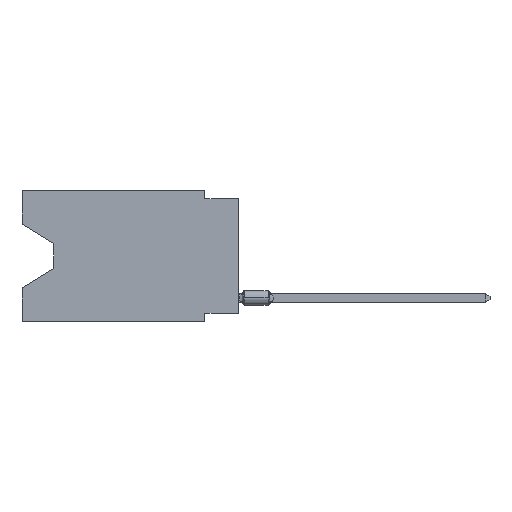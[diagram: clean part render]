
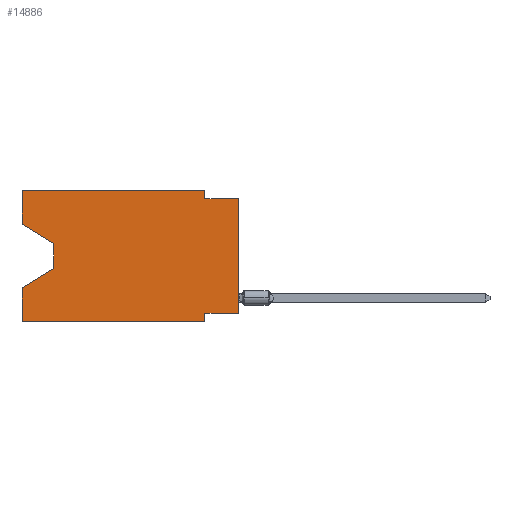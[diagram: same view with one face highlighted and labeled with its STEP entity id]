
A CAD part, left-side view. The second image highlights one B-rep face of the part: STEP entity #14886.
In plain terms, the highlighted planar face has unit normal (-1, 0, 0).
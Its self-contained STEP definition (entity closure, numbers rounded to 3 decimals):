
#68 = CARTESIAN_POINT ( 'NONE',  ( 0., 16.383, 0. ) ) ;
#351 = ORIENTED_EDGE ( 'NONE', *, *, #17122, .T. ) ;
#352 = DIRECTION ( 'NONE',  ( 0., -1., 0. ) ) ;
#699 = DIRECTION ( 'NONE',  ( 1., 0., 0. ) ) ;
#1004 = LINE ( 'NONE', #1097, #1624 ) ;
#1097 = CARTESIAN_POINT ( 'NONE',  ( 0., 2.54, 0. ) ) ;
#1304 = CARTESIAN_POINT ( 'NONE',  ( 0., 16.383, -2.546 ) ) ;
#1529 = CARTESIAN_POINT ( 'NONE',  ( 0., 2.54, -9.271 ) ) ;
#1624 = VECTOR ( 'NONE', #12020, 1000. ) ;
#1640 = CARTESIAN_POINT ( 'NONE',  ( 0., 0., -9.271 ) ) ;
#2040 = LINE ( 'NONE', #15904, #15193 ) ;
#2059 = VERTEX_POINT ( 'NONE', #4552 ) ;
#2344 = CARTESIAN_POINT ( 'NONE',  ( 0., 13.97, -5.893 ) ) ;
#2637 = VERTEX_POINT ( 'NONE', #11923 ) ;
#2653 = DIRECTION ( 'NONE',  ( 0., 0., 1. ) ) ;
#2704 = CARTESIAN_POINT ( 'NONE',  ( 0., 13.97, -5.893 ) ) ;
#2888 = VECTOR ( 'NONE', #3939, 1000. ) ;
#2911 = VERTEX_POINT ( 'NONE', #11266 ) ;
#3112 = EDGE_CURVE ( 'NONE', #11366, #15865, #9222, .T. ) ;
#3512 = VECTOR ( 'NONE', #2653, 1000. ) ;
#3543 = LINE ( 'NONE', #2344, #10102 ) ;
#3648 = ORIENTED_EDGE ( 'NONE', *, *, #13792, .T. ) ;
#3939 = DIRECTION ( 'NONE',  ( 0., 0., -1. ) ) ;
#4046 = CARTESIAN_POINT ( 'NONE',  ( 0., 0., 0. ) ) ;
#4280 = EDGE_CURVE ( 'NONE', #17562, #2059, #11277, .T. ) ;
#4552 = CARTESIAN_POINT ( 'NONE',  ( 0., 2.54, 0. ) ) ;
#4559 = VECTOR ( 'NONE', #352, 1000. ) ;
#4783 = EDGE_CURVE ( 'NONE', #11562, #2637, #3543, .T. ) ;
#5107 = VECTOR ( 'NONE', #10067, 1000. ) ;
#5238 = PLANE ( 'NONE',  #9570 ) ;
#5374 = LINE ( 'NONE', #1304, #11021 ) ;
#5442 = CARTESIAN_POINT ( 'NONE',  ( 0., 0., -0.635 ) ) ;
#5646 = VECTOR ( 'NONE', #7770, 1000. ) ;
#6226 = DIRECTION ( 'NONE',  ( 0., 0.855, -0.519 ) ) ;
#6494 = VERTEX_POINT ( 'NONE', #14141 ) ;
#6963 = EDGE_CURVE ( 'NONE', #7016, #17491, #8126, .T. ) ;
#7016 = VERTEX_POINT ( 'NONE', #1640 ) ;
#7262 = VECTOR ( 'NONE', #18008, 1000. ) ;
#7550 = ORIENTED_EDGE ( 'NONE', *, *, #3112, .F. ) ;
#7770 = DIRECTION ( 'NONE',  ( 0., -1., 0. ) ) ;
#8126 = LINE ( 'NONE', #4046, #7262 ) ;
#8236 = ORIENTED_EDGE ( 'NONE', *, *, #13847, .F. ) ;
#8739 = VERTEX_POINT ( 'NONE', #11519 ) ;
#8771 = ORIENTED_EDGE ( 'NONE', *, *, #13661, .F. ) ;
#9021 = EDGE_LOOP ( 'NONE', ( #351, #3648, #15853, #8771, #10507, #7550, #16704, #13132, #16457, #8236, #15598, #14436 ) ) ;
#9061 = LINE ( 'NONE', #14797, #4559 ) ;
#9222 = LINE ( 'NONE', #9313, #2888 ) ;
#9313 = CARTESIAN_POINT ( 'NONE',  ( 0., 2.54, -9.906 ) ) ;
#9332 = CARTESIAN_POINT ( 'NONE',  ( 0., 13.97, -4.013 ) ) ;
#9506 = LINE ( 'NONE', #9332, #14004 ) ;
#9570 = AXIS2_PLACEMENT_3D ( 'NONE', #11996, #699, #10512 ) ;
#9881 = LINE ( 'NONE', #14230, #14879 ) ;
#10067 = DIRECTION ( 'NONE',  ( 0., -1., 0. ) ) ;
#10102 = VECTOR ( 'NONE', #6226, 1000. ) ;
#10199 = EDGE_CURVE ( 'NONE', #2911, #17562, #16982, .T. ) ;
#10507 = ORIENTED_EDGE ( 'NONE', *, *, #13649, .T. ) ;
#10512 = DIRECTION ( 'NONE',  ( 0., 0., -1. ) ) ;
#10697 = FACE_OUTER_BOUND ( 'NONE', #9021, .T. ) ;
#10812 = DIRECTION ( 'NONE',  ( 0., 0., -1. ) ) ;
#10987 = CARTESIAN_POINT ( 'NONE',  ( 0., 2.54, -9.906 ) ) ;
#11019 = DIRECTION ( 'NONE',  ( 0., -0.855, -0.519 ) ) ;
#11021 = VECTOR ( 'NONE', #11019, 1000. ) ;
#11266 = CARTESIAN_POINT ( 'NONE',  ( 0., 16.383, -2.546 ) ) ;
#11277 = LINE ( 'NONE', #15624, #5107 ) ;
#11366 = VERTEX_POINT ( 'NONE', #1529 ) ;
#11507 = VERTEX_POINT ( 'NONE', #12151 ) ;
#11519 = CARTESIAN_POINT ( 'NONE',  ( 0., 2.54, -0.635 ) ) ;
#11562 = VERTEX_POINT ( 'NONE', #2704 ) ;
#11923 = CARTESIAN_POINT ( 'NONE',  ( 0., 16.383, -7.36 ) ) ;
#11996 = CARTESIAN_POINT ( 'NONE',  ( 0., 16.383, 0. ) ) ;
#12020 = DIRECTION ( 'NONE',  ( 0., 0., -1. ) ) ;
#12151 = CARTESIAN_POINT ( 'NONE',  ( 0., 16.383, -9.906 ) ) ;
#12233 = EDGE_CURVE ( 'NONE', #8739, #17491, #14605, .T. ) ;
#13132 = ORIENTED_EDGE ( 'NONE', *, *, #6963, .T. ) ;
#13649 = EDGE_CURVE ( 'NONE', #11507, #15865, #9061, .T. ) ;
#13661 = EDGE_CURVE ( 'NONE', #11507, #2637, #2040, .T. ) ;
#13792 = EDGE_CURVE ( 'NONE', #6494, #11562, #9506, .T. ) ;
#13847 = EDGE_CURVE ( 'NONE', #2059, #8739, #1004, .T. ) ;
#14004 = VECTOR ( 'NONE', #10812, 1000. ) ;
#14141 = CARTESIAN_POINT ( 'NONE',  ( 0., 13.97, -4.013 ) ) ;
#14208 = CARTESIAN_POINT ( 'NONE',  ( 0., 16.383, 0. ) ) ;
#14230 = CARTESIAN_POINT ( 'NONE',  ( 0., 0., -9.271 ) ) ;
#14436 = ORIENTED_EDGE ( 'NONE', *, *, #10199, .F. ) ;
#14605 = LINE ( 'NONE', #17382, #5646 ) ;
#14797 = CARTESIAN_POINT ( 'NONE',  ( 0., 16.383, -9.906 ) ) ;
#14879 = VECTOR ( 'NONE', #16909, 1000. ) ;
#14886 = ADVANCED_FACE ( 'NONE', ( #10697 ), #5238, .F. ) ;
#15193 = VECTOR ( 'NONE', #15996, 1000. ) ;
#15598 = ORIENTED_EDGE ( 'NONE', *, *, #4280, .F. ) ;
#15624 = CARTESIAN_POINT ( 'NONE',  ( 0., 16.383, 0. ) ) ;
#15853 = ORIENTED_EDGE ( 'NONE', *, *, #4783, .T. ) ;
#15865 = VERTEX_POINT ( 'NONE', #10987 ) ;
#15904 = CARTESIAN_POINT ( 'NONE',  ( 0., 16.383, 0. ) ) ;
#15996 = DIRECTION ( 'NONE',  ( 0., 0., 1. ) ) ;
#16457 = ORIENTED_EDGE ( 'NONE', *, *, #12233, .F. ) ;
#16704 = ORIENTED_EDGE ( 'NONE', *, *, #17672, .F. ) ;
#16909 = DIRECTION ( 'NONE',  ( 0., 1., 0. ) ) ;
#16982 = LINE ( 'NONE', #14208, #3512 ) ;
#17122 = EDGE_CURVE ( 'NONE', #2911, #6494, #5374, .T. ) ;
#17382 = CARTESIAN_POINT ( 'NONE',  ( 0., 0., -0.635 ) ) ;
#17491 = VERTEX_POINT ( 'NONE', #5442 ) ;
#17562 = VERTEX_POINT ( 'NONE', #68 ) ;
#17672 = EDGE_CURVE ( 'NONE', #7016, #11366, #9881, .T. ) ;
#18008 = DIRECTION ( 'NONE',  ( 0., 0., 1. ) ) ;
